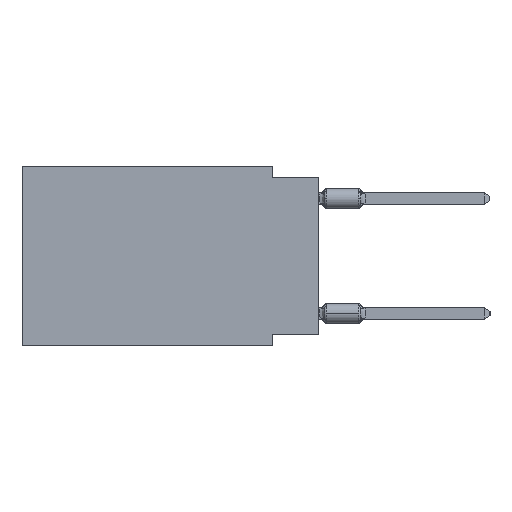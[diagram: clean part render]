
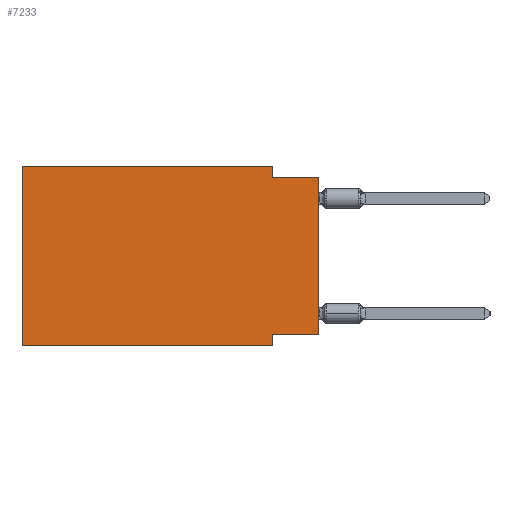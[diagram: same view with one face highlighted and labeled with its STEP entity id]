
A CAD part, left-side view. The second image highlights one B-rep face of the part: STEP entity #7233.
In plain terms, the highlighted planar face has unit normal (-1, 0, 0).
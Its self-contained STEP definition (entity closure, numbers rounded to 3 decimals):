
#94 = LINE ( 'NONE', #27285, #28294 ) ;
#214 = EDGE_CURVE ( 'NONE', #13241, #13790, #11386, .T. ) ;
#700 = CARTESIAN_POINT ( 'NONE',  ( 0., 16.383, 0. ) ) ;
#1667 = CARTESIAN_POINT ( 'NONE',  ( 0., 0., -9.271 ) ) ;
#1867 = ORIENTED_EDGE ( 'NONE', *, *, #25996, .F. ) ;
#2113 = ORIENTED_EDGE ( 'NONE', *, *, #3922, .T. ) ;
#2248 = CARTESIAN_POINT ( 'NONE',  ( 0., 2.54, 0. ) ) ;
#2652 = ORIENTED_EDGE ( 'NONE', *, *, #22445, .F. ) ;
#3819 = ORIENTED_EDGE ( 'NONE', *, *, #5016, .F. ) ;
#3844 = ORIENTED_EDGE ( 'NONE', *, *, #14220, .F. ) ;
#3922 = EDGE_CURVE ( 'NONE', #12495, #17063, #22246, .T. ) ;
#4706 = DIRECTION ( 'NONE',  ( 0., -1., 0. ) ) ;
#4982 = VECTOR ( 'NONE', #18627, 1000. ) ;
#5016 = EDGE_CURVE ( 'NONE', #17508, #17063, #94, .T. ) ;
#5566 = CARTESIAN_POINT ( 'NONE',  ( 0., 16.383, -9.906 ) ) ;
#5876 = AXIS2_PLACEMENT_3D ( 'NONE', #700, #16501, #11064 ) ;
#7233 = ADVANCED_FACE ( 'NONE', ( #21439 ), #31344, .F. ) ;
#8519 = DIRECTION ( 'NONE',  ( 0., -1., 0. ) ) ;
#9171 = ORIENTED_EDGE ( 'NONE', *, *, #10501, .F. ) ;
#9800 = CARTESIAN_POINT ( 'NONE',  ( 0., 16.383, 0. ) ) ;
#10214 = CARTESIAN_POINT ( 'NONE',  ( 0., 2.54, -9.906 ) ) ;
#10501 = EDGE_CURVE ( 'NONE', #13790, #10993, #31742, .T. ) ;
#10993 = VERTEX_POINT ( 'NONE', #29880 ) ;
#11064 = DIRECTION ( 'NONE',  ( 0., 0., -1. ) ) ;
#11386 = LINE ( 'NONE', #16013, #20818 ) ;
#12495 = VERTEX_POINT ( 'NONE', #1667 ) ;
#12638 = VERTEX_POINT ( 'NONE', #10214 ) ;
#13196 = EDGE_CURVE ( 'NONE', #13241, #12638, #30955, .T. ) ;
#13241 = VERTEX_POINT ( 'NONE', #5566 ) ;
#13790 = VERTEX_POINT ( 'NONE', #14535 ) ;
#14220 = EDGE_CURVE ( 'NONE', #12495, #26550, #25692, .T. ) ;
#14509 = CARTESIAN_POINT ( 'NONE',  ( 0., 0., 0. ) ) ;
#14535 = CARTESIAN_POINT ( 'NONE',  ( 0., 16.383, 0. ) ) ;
#15323 = ORIENTED_EDGE ( 'NONE', *, *, #214, .F. ) ;
#15994 = LINE ( 'NONE', #16157, #4982 ) ;
#16013 = CARTESIAN_POINT ( 'NONE',  ( 0., 16.383, 0. ) ) ;
#16157 = CARTESIAN_POINT ( 'NONE',  ( 0., 2.54, -9.906 ) ) ;
#16399 = VECTOR ( 'NONE', #28011, 1000. ) ;
#16501 = DIRECTION ( 'NONE',  ( 1., 0., 0. ) ) ;
#17063 = VERTEX_POINT ( 'NONE', #29642 ) ;
#17345 = VECTOR ( 'NONE', #24235, 1000. ) ;
#17508 = VERTEX_POINT ( 'NONE', #26456 ) ;
#18572 = ORIENTED_EDGE ( 'NONE', *, *, #13196, .T. ) ;
#18581 = CARTESIAN_POINT ( 'NONE',  ( 0., 16.383, -9.906 ) ) ;
#18627 = DIRECTION ( 'NONE',  ( 0., 0., -1. ) ) ;
#20575 = CARTESIAN_POINT ( 'NONE',  ( 0., 0., -9.271 ) ) ;
#20818 = VECTOR ( 'NONE', #25904, 1000. ) ;
#21439 = FACE_OUTER_BOUND ( 'NONE', #25146, .T. ) ;
#22246 = LINE ( 'NONE', #14509, #17345 ) ;
#22350 = DIRECTION ( 'NONE',  ( 0., 0., -1. ) ) ;
#22445 = EDGE_CURVE ( 'NONE', #26550, #12638, #15994, .T. ) ;
#24235 = DIRECTION ( 'NONE',  ( 0., 0., 1. ) ) ;
#24647 = DIRECTION ( 'NONE',  ( 0., -1., 0. ) ) ;
#24832 = LINE ( 'NONE', #2248, #27561 ) ;
#25146 = EDGE_LOOP ( 'NONE', ( #2113, #3819, #1867, #9171, #15323, #18572, #2652, #3844 ) ) ;
#25692 = LINE ( 'NONE', #20575, #16399 ) ;
#25904 = DIRECTION ( 'NONE',  ( 0., 0., 1. ) ) ;
#25996 = EDGE_CURVE ( 'NONE', #10993, #17508, #24832, .T. ) ;
#26456 = CARTESIAN_POINT ( 'NONE',  ( 0., 2.54, -0.635 ) ) ;
#26550 = VERTEX_POINT ( 'NONE', #31033 ) ;
#26635 = VECTOR ( 'NONE', #24647, 1000. ) ;
#27285 = CARTESIAN_POINT ( 'NONE',  ( 0., 0., -0.635 ) ) ;
#27401 = VECTOR ( 'NONE', #8519, 1000. ) ;
#27561 = VECTOR ( 'NONE', #22350, 1000. ) ;
#28011 = DIRECTION ( 'NONE',  ( 0., 1., 0. ) ) ;
#28294 = VECTOR ( 'NONE', #4706, 1000. ) ;
#29642 = CARTESIAN_POINT ( 'NONE',  ( 0., 0., -0.635 ) ) ;
#29880 = CARTESIAN_POINT ( 'NONE',  ( 0., 2.54, 0. ) ) ;
#30955 = LINE ( 'NONE', #18581, #27401 ) ;
#31033 = CARTESIAN_POINT ( 'NONE',  ( 0., 2.54, -9.271 ) ) ;
#31344 = PLANE ( 'NONE',  #5876 ) ;
#31742 = LINE ( 'NONE', #9800, #26635 ) ;
